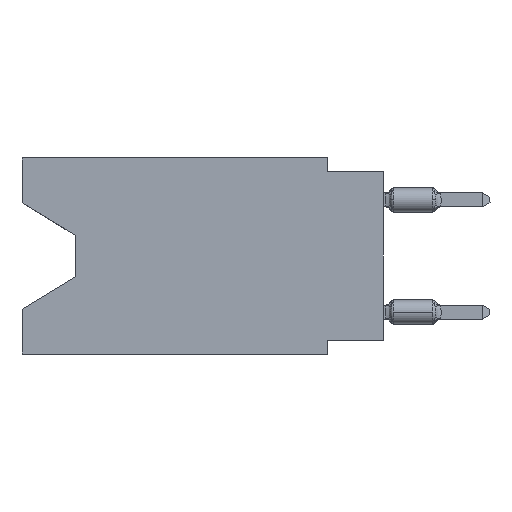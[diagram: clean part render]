
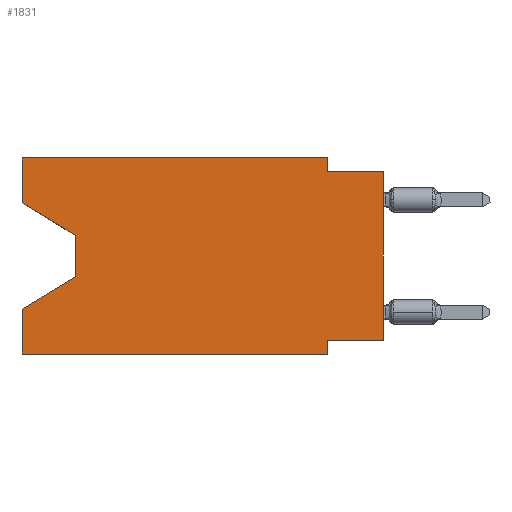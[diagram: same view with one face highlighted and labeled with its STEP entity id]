
A CAD part, left-side view. The second image highlights one B-rep face of the part: STEP entity #1831.
In plain terms, the highlighted planar face has unit normal (-1, 0, 0).
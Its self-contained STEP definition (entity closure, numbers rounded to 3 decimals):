
#586 = CARTESIAN_POINT ( 'NONE',  ( 0., 16.383, 0. ) ) ;
#902 = ORIENTED_EDGE ( 'NONE', *, *, #6160, .F. ) ;
#949 = LINE ( 'NONE', #18238, #2368 ) ;
#1068 = CARTESIAN_POINT ( 'NONE',  ( 0., 2.54, -0.635 ) ) ;
#1205 = ORIENTED_EDGE ( 'NONE', *, *, #17836, .T. ) ;
#1606 = DIRECTION ( 'NONE',  ( 0., 0., -1. ) ) ;
#1831 = ADVANCED_FACE ( 'NONE', ( #15254 ), #15442, .F. ) ;
#1944 = VERTEX_POINT ( 'NONE', #9864 ) ;
#2368 = VECTOR ( 'NONE', #11192, 1000. ) ;
#2869 = VECTOR ( 'NONE', #17281, 1000. ) ;
#2893 = DIRECTION ( 'NONE',  ( 0., 0., -1. ) ) ;
#2927 = VERTEX_POINT ( 'NONE', #3394 ) ;
#3157 = VERTEX_POINT ( 'NONE', #1068 ) ;
#3394 = CARTESIAN_POINT ( 'NONE',  ( 0., 0., -8.255 ) ) ;
#3673 = ORIENTED_EDGE ( 'NONE', *, *, #10697, .F. ) ;
#3715 = CARTESIAN_POINT ( 'NONE',  ( 0., 16.383, 0. ) ) ;
#3904 = ORIENTED_EDGE ( 'NONE', *, *, #12270, .T. ) ;
#4001 = VECTOR ( 'NONE', #14563, 1000. ) ;
#4184 = DIRECTION ( 'NONE',  ( 1., 0., 0. ) ) ;
#4385 = EDGE_CURVE ( 'NONE', #2927, #15116, #8800, .T. ) ;
#4402 = CARTESIAN_POINT ( 'NONE',  ( 0., 16.383, -8.89 ) ) ;
#4619 = DIRECTION ( 'NONE',  ( 0., 0., -1. ) ) ;
#4771 = VERTEX_POINT ( 'NONE', #10255 ) ;
#5284 = CARTESIAN_POINT ( 'NONE',  ( 0., 16.383, 0. ) ) ;
#5306 = ORIENTED_EDGE ( 'NONE', *, *, #9606, .F. ) ;
#5404 = EDGE_CURVE ( 'NONE', #17192, #17724, #9464, .T. ) ;
#5650 = EDGE_CURVE ( 'NONE', #8490, #16742, #17606, .T. ) ;
#5714 = EDGE_CURVE ( 'NONE', #8490, #11983, #949, .T. ) ;
#6160 = EDGE_CURVE ( 'NONE', #16742, #8512, #15067, .T. ) ;
#6912 = VECTOR ( 'NONE', #4619, 1000. ) ;
#6975 = DIRECTION ( 'NONE',  ( 0., -1., 0. ) ) ;
#7091 = CARTESIAN_POINT ( 'NONE',  ( 0., 0., -8.255 ) ) ;
#7346 = CARTESIAN_POINT ( 'NONE',  ( 0., 0., -0.635 ) ) ;
#7567 = LINE ( 'NONE', #15954, #4001 ) ;
#7999 = CARTESIAN_POINT ( 'NONE',  ( 0., 2.54, 0. ) ) ;
#8490 = VERTEX_POINT ( 'NONE', #14704 ) ;
#8512 = VERTEX_POINT ( 'NONE', #7999 ) ;
#8800 = LINE ( 'NONE', #11584, #12363 ) ;
#9064 = DIRECTION ( 'NONE',  ( 0., -1., 0. ) ) ;
#9157 = CARTESIAN_POINT ( 'NONE',  ( 0., 16.383, -8.89 ) ) ;
#9330 = AXIS2_PLACEMENT_3D ( 'NONE', #11267, #4184, #2893 ) ;
#9442 = CARTESIAN_POINT ( 'NONE',  ( 0., 13.97, -3.505 ) ) ;
#9464 = LINE ( 'NONE', #5284, #12494 ) ;
#9606 = EDGE_CURVE ( 'NONE', #8512, #3157, #15643, .T. ) ;
#9696 = DIRECTION ( 'NONE',  ( 0., 1., 0. ) ) ;
#9739 = VECTOR ( 'NONE', #9696, 1000. ) ;
#9864 = CARTESIAN_POINT ( 'NONE',  ( 0., 2.54, -8.255 ) ) ;
#9933 = VERTEX_POINT ( 'NONE', #10055 ) ;
#10055 = CARTESIAN_POINT ( 'NONE',  ( 0., 2.54, -8.89 ) ) ;
#10143 = ORIENTED_EDGE ( 'NONE', *, *, #10880, .F. ) ;
#10163 = LINE ( 'NONE', #14615, #11535 ) ;
#10255 = CARTESIAN_POINT ( 'NONE',  ( 0., 13.97, -5.385 ) ) ;
#10552 = LINE ( 'NONE', #9157, #17612 ) ;
#10697 = EDGE_CURVE ( 'NONE', #2927, #1944, #14065, .T. ) ;
#10880 = EDGE_CURVE ( 'NONE', #1944, #9933, #10163, .T. ) ;
#10898 = ORIENTED_EDGE ( 'NONE', *, *, #18382, .T. ) ;
#11192 = DIRECTION ( 'NONE',  ( 0., -0.855, -0.519 ) ) ;
#11267 = CARTESIAN_POINT ( 'NONE',  ( 0., 16.383, 0. ) ) ;
#11274 = ORIENTED_EDGE ( 'NONE', *, *, #5650, .F. ) ;
#11535 = VECTOR ( 'NONE', #11560, 1000. ) ;
#11560 = DIRECTION ( 'NONE',  ( 0., 0., -1. ) ) ;
#11584 = CARTESIAN_POINT ( 'NONE',  ( 0., 0., 0. ) ) ;
#11611 = CARTESIAN_POINT ( 'NONE',  ( 0., 13.97, -3.505 ) ) ;
#11983 = VERTEX_POINT ( 'NONE', #9442 ) ;
#12270 = EDGE_CURVE ( 'NONE', #4771, #17724, #7567, .T. ) ;
#12363 = VECTOR ( 'NONE', #14378, 1000. ) ;
#12494 = VECTOR ( 'NONE', #13939, 1000. ) ;
#13003 = CARTESIAN_POINT ( 'NONE',  ( 0., 16.383, 0. ) ) ;
#13492 = VECTOR ( 'NONE', #6975, 1000. ) ;
#13701 = ORIENTED_EDGE ( 'NONE', *, *, #5404, .F. ) ;
#13939 = DIRECTION ( 'NONE',  ( 0., 0., 1. ) ) ;
#14030 = LINE ( 'NONE', #7346, #2869 ) ;
#14055 = ORIENTED_EDGE ( 'NONE', *, *, #15038, .F. ) ;
#14065 = LINE ( 'NONE', #7091, #9739 ) ;
#14215 = LINE ( 'NONE', #11611, #6912 ) ;
#14378 = DIRECTION ( 'NONE',  ( 0., 0., 1. ) ) ;
#14448 = CARTESIAN_POINT ( 'NONE',  ( 0., 2.54, 0. ) ) ;
#14563 = DIRECTION ( 'NONE',  ( 0., 0.855, -0.519 ) ) ;
#14615 = CARTESIAN_POINT ( 'NONE',  ( 0., 2.54, -8.89 ) ) ;
#14668 = CARTESIAN_POINT ( 'NONE',  ( 0., 0., -0.635 ) ) ;
#14704 = CARTESIAN_POINT ( 'NONE',  ( 0., 16.383, -2.038 ) ) ;
#14941 = ORIENTED_EDGE ( 'NONE', *, *, #5714, .T. ) ;
#15038 = EDGE_CURVE ( 'NONE', #3157, #15116, #14030, .T. ) ;
#15067 = LINE ( 'NONE', #3715, #13492 ) ;
#15116 = VERTEX_POINT ( 'NONE', #14668 ) ;
#15254 = FACE_OUTER_BOUND ( 'NONE', #18034, .T. ) ;
#15351 = VECTOR ( 'NONE', #1606, 1000. ) ;
#15398 = ORIENTED_EDGE ( 'NONE', *, *, #4385, .T. ) ;
#15442 = PLANE ( 'NONE',  #9330 ) ;
#15643 = LINE ( 'NONE', #14448, #15351 ) ;
#15954 = CARTESIAN_POINT ( 'NONE',  ( 0., 13.97, -5.385 ) ) ;
#16088 = CARTESIAN_POINT ( 'NONE',  ( 0., 16.383, -6.852 ) ) ;
#16486 = DIRECTION ( 'NONE',  ( 0., 0., 1. ) ) ;
#16742 = VERTEX_POINT ( 'NONE', #13003 ) ;
#16943 = VECTOR ( 'NONE', #16486, 1000. ) ;
#17192 = VERTEX_POINT ( 'NONE', #4402 ) ;
#17281 = DIRECTION ( 'NONE',  ( 0., -1., 0. ) ) ;
#17606 = LINE ( 'NONE', #586, #16943 ) ;
#17612 = VECTOR ( 'NONE', #9064, 1000. ) ;
#17724 = VERTEX_POINT ( 'NONE', #16088 ) ;
#17836 = EDGE_CURVE ( 'NONE', #11983, #4771, #14215, .T. ) ;
#18034 = EDGE_LOOP ( 'NONE', ( #14941, #1205, #3904, #13701, #10898, #10143, #3673, #15398, #14055, #5306, #902, #11274 ) ) ;
#18238 = CARTESIAN_POINT ( 'NONE',  ( 0., 16.383, -2.038 ) ) ;
#18382 = EDGE_CURVE ( 'NONE', #17192, #9933, #10552, .T. ) ;
